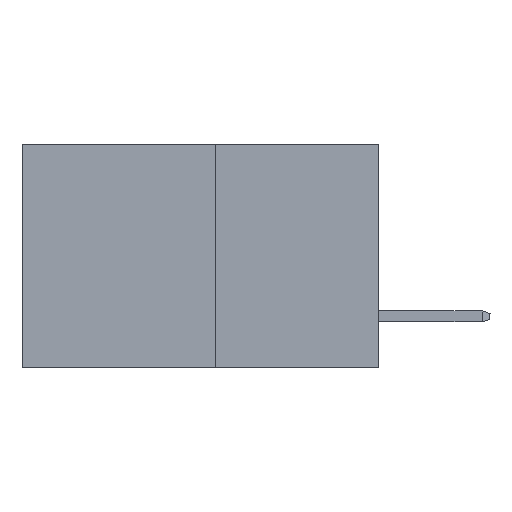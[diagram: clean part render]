
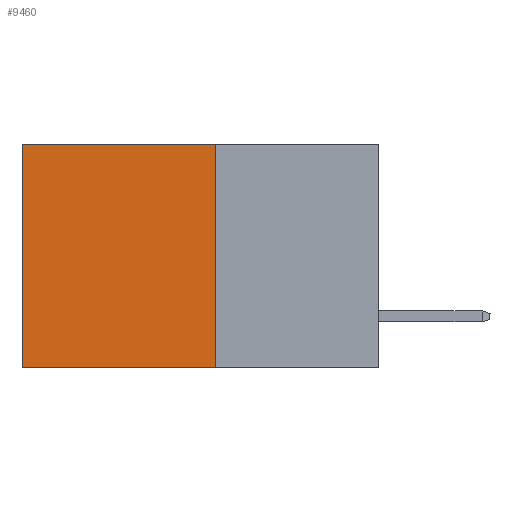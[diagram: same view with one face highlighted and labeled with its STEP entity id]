
A CAD part, left-side view. The second image highlights one B-rep face of the part: STEP entity #9460.
In plain terms, the highlighted planar face has unit normal (-1, 0, 0).
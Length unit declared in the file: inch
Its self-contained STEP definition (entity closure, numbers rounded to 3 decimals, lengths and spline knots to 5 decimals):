
#2949 = ORIENTED_EDGE ( 'NONE', *, *, #13915, .T. ) ;
#3474 = LINE ( 'NONE', #7824, #16127 ) ;
#3522 = VECTOR ( 'NONE', #13748, 39.37008 ) ;
#3926 = LINE ( 'NONE', #7552, #3522 ) ;
#4312 = FACE_OUTER_BOUND ( 'NONE', #15447, .T. ) ;
#4536 = VECTOR ( 'NONE', #12767, 39.37008 ) ;
#5448 = CARTESIAN_POINT ( 'NONE',  ( 0.277, 0.27, -0.37 ) ) ;
#5914 = ORIENTED_EDGE ( 'NONE', *, *, #9247, .F. ) ;
#6008 = VECTOR ( 'NONE', #14254, 39.37008 ) ;
#6432 = LINE ( 'NONE', #5448, #6008 ) ;
#7304 = ORIENTED_EDGE ( 'NONE', *, *, #13764, .F. ) ;
#7552 = CARTESIAN_POINT ( 'NONE',  ( 0.277, 0.59, -0.37 ) ) ;
#7556 = DIRECTION ( 'NONE',  ( 0., 1., 0. ) ) ;
#7821 = VERTEX_POINT ( 'NONE', #10518 ) ;
#7824 = CARTESIAN_POINT ( 'NONE',  ( 0.277, 0.27, 0. ) ) ;
#8024 = CARTESIAN_POINT ( 'NONE',  ( 0.277, 0.27, 0. ) ) ;
#8453 = VERTEX_POINT ( 'NONE', #8024 ) ;
#8511 = CARTESIAN_POINT ( 'NONE',  ( 0.277, 0.59, -0.37 ) ) ;
#9247 = EDGE_CURVE ( 'NONE', #15143, #14893, #14233, .T. ) ;
#9460 = ADVANCED_FACE ( 'NONE', ( #4312 ), #11206, .F. ) ;
#9927 = EDGE_CURVE ( 'NONE', #8453, #7821, #3474, .T. ) ;
#10461 = ORIENTED_EDGE ( 'NONE', *, *, #9927, .T. ) ;
#10518 = CARTESIAN_POINT ( 'NONE',  ( 0.277, 0.59, 0. ) ) ;
#11124 = DIRECTION ( 'NONE',  ( 0., 0., -1. ) ) ;
#11127 = DIRECTION ( 'NONE',  ( 1., 0., 0. ) ) ;
#11159 = CARTESIAN_POINT ( 'NONE',  ( 0.277, 0.27, -0.37 ) ) ;
#11206 = PLANE ( 'NONE',  #13812 ) ;
#12622 = CARTESIAN_POINT ( 'NONE',  ( 0.277, 0.27, -0.37 ) ) ;
#12767 = DIRECTION ( 'NONE',  ( 0., 1., 0. ) ) ;
#12784 = CARTESIAN_POINT ( 'NONE',  ( 0.277, 0.27, -0.37 ) ) ;
#13748 = DIRECTION ( 'NONE',  ( 0., 0., -1. ) ) ;
#13764 = EDGE_CURVE ( 'NONE', #8453, #15143, #6432, .T. ) ;
#13812 = AXIS2_PLACEMENT_3D ( 'NONE', #11159, #11127, #11124 ) ;
#13915 = EDGE_CURVE ( 'NONE', #7821, #14893, #3926, .T. ) ;
#14233 = LINE ( 'NONE', #12784, #4536 ) ;
#14254 = DIRECTION ( 'NONE',  ( 0., 0., -1. ) ) ;
#14893 = VERTEX_POINT ( 'NONE', #8511 ) ;
#15143 = VERTEX_POINT ( 'NONE', #12622 ) ;
#15447 = EDGE_LOOP ( 'NONE', ( #2949, #5914, #7304, #10461 ) ) ;
#16127 = VECTOR ( 'NONE', #7556, 39.37008 ) ;
